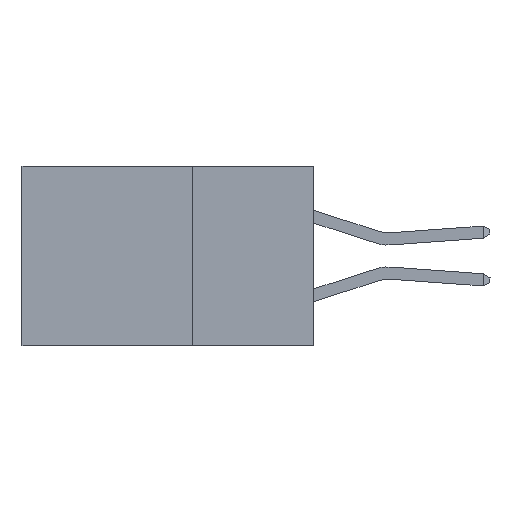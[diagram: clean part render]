
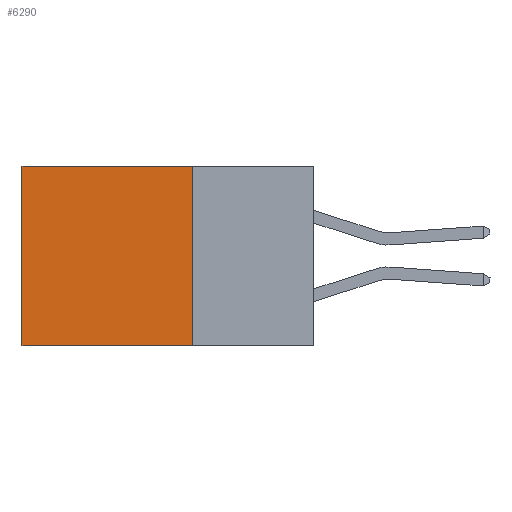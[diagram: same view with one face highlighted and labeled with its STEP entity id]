
A CAD part, left-side view. The second image highlights one B-rep face of the part: STEP entity #6290.
In plain terms, the highlighted planar face has unit normal (-1, 0, 0).
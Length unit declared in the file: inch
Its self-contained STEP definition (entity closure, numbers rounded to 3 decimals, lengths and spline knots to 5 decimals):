
#760 = VERTEX_POINT ( 'NONE', #29191 ) ;
#2814 = DIRECTION ( 'NONE',  ( 0., 1., 0. ) ) ;
#4687 = LINE ( 'NONE', #21361, #12219 ) ;
#6290 = ADVANCED_FACE ( 'NONE', ( #32805 ), #7874, .F. ) ;
#6642 = DIRECTION ( 'NONE',  ( 0., 0., -1. ) ) ;
#7874 = PLANE ( 'NONE',  #22917 ) ;
#8342 = EDGE_CURVE ( 'NONE', #16342, #11351, #25235, .T. ) ;
#10750 = EDGE_LOOP ( 'NONE', ( #21075, #34216, #25485, #15015 ) ) ;
#11351 = VERTEX_POINT ( 'NONE', #12681 ) ;
#12011 = LINE ( 'NONE', #22957, #34589 ) ;
#12219 = VECTOR ( 'NONE', #18647, 39.37008 ) ;
#12681 = CARTESIAN_POINT ( 'NONE',  ( 0.2875, 0.6, -0.37 ) ) ;
#15015 = ORIENTED_EDGE ( 'NONE', *, *, #18959, .T. ) ;
#16342 = VERTEX_POINT ( 'NONE', #30341 ) ;
#16596 = LINE ( 'NONE', #22181, #25938 ) ;
#17691 = VERTEX_POINT ( 'NONE', #32782 ) ;
#18622 = DIRECTION ( 'NONE',  ( 1., 0., 0. ) ) ;
#18647 = DIRECTION ( 'NONE',  ( 0., 1., 0. ) ) ;
#18959 = EDGE_CURVE ( 'NONE', #760, #16342, #4687, .T. ) ;
#19144 = CARTESIAN_POINT ( 'NONE',  ( 0.2875, 0.25, 0. ) ) ;
#19295 = EDGE_CURVE ( 'NONE', #760, #17691, #12011, .T. ) ;
#20186 = DIRECTION ( 'NONE',  ( 0., 0., -1. ) ) ;
#21075 = ORIENTED_EDGE ( 'NONE', *, *, #8342, .T. ) ;
#21361 = CARTESIAN_POINT ( 'NONE',  ( 0.2875, 0.25, 0. ) ) ;
#21851 = VECTOR ( 'NONE', #20186, 39.37008 ) ;
#22181 = CARTESIAN_POINT ( 'NONE',  ( 0.2875, 0.25, -0.37 ) ) ;
#22917 = AXIS2_PLACEMENT_3D ( 'NONE', #19144, #18622, #24022 ) ;
#22957 = CARTESIAN_POINT ( 'NONE',  ( 0.2875, 0.25, 0. ) ) ;
#24022 = DIRECTION ( 'NONE',  ( 0., 0., -1. ) ) ;
#24888 = CARTESIAN_POINT ( 'NONE',  ( 0.2875, 0.6, 0. ) ) ;
#25235 = LINE ( 'NONE', #24888, #21851 ) ;
#25485 = ORIENTED_EDGE ( 'NONE', *, *, #19295, .F. ) ;
#25938 = VECTOR ( 'NONE', #2814, 39.37008 ) ;
#29191 = CARTESIAN_POINT ( 'NONE',  ( 0.2875, 0.25, 0. ) ) ;
#30341 = CARTESIAN_POINT ( 'NONE',  ( 0.2875, 0.6, 0. ) ) ;
#32469 = EDGE_CURVE ( 'NONE', #17691, #11351, #16596, .T. ) ;
#32782 = CARTESIAN_POINT ( 'NONE',  ( 0.2875, 0.25, -0.37 ) ) ;
#32805 = FACE_OUTER_BOUND ( 'NONE', #10750, .T. ) ;
#34216 = ORIENTED_EDGE ( 'NONE', *, *, #32469, .F. ) ;
#34589 = VECTOR ( 'NONE', #6642, 39.37008 ) ;
